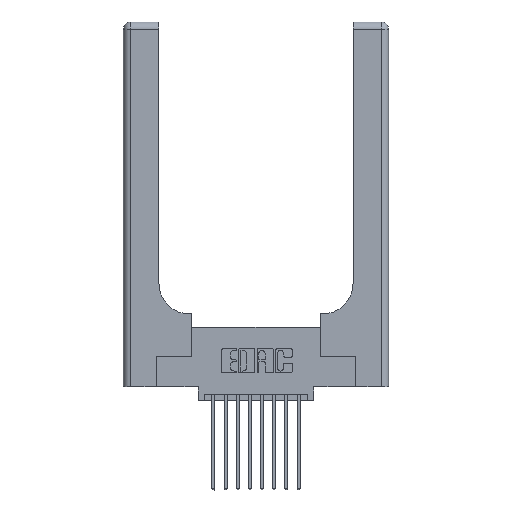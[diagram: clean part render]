
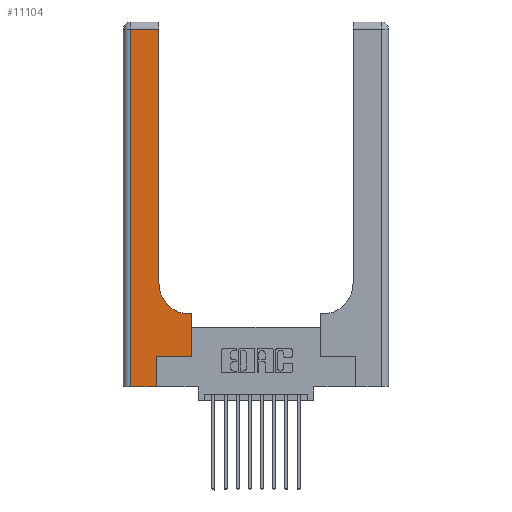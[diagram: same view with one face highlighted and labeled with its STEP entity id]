
A CAD part, top view. The second image highlights one B-rep face of the part: STEP entity #11104.
In plain terms, the highlighted planar face has unit normal (0, 0, 1).
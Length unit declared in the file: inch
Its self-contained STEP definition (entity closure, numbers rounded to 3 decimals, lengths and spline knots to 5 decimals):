
#32 = DIRECTION ( 'NONE',  ( -1., 0., 0. ) ) ;
#150 = DIRECTION ( 'NONE',  ( 0., 1., 0. ) ) ;
#166 = VERTEX_POINT ( 'NONE', #7051 ) ;
#197 = VECTOR ( 'NONE', #150, 39.37008 ) ;
#571 = VERTEX_POINT ( 'NONE', #14026 ) ;
#918 = EDGE_CURVE ( 'NONE', #5515, #571, #5145, .T. ) ;
#1034 = VERTEX_POINT ( 'NONE', #2276 ) ;
#1112 = EDGE_CURVE ( 'NONE', #11790, #7345, #11933, .T. ) ;
#1241 = CARTESIAN_POINT ( 'NONE',  ( 0.2915, 0.6, 0.37 ) ) ;
#1293 = VECTOR ( 'NONE', #6406, 39.37008 ) ;
#1308 = EDGE_CURVE ( 'NONE', #15248, #11790, #1382, .T. ) ;
#1382 = LINE ( 'NONE', #6415, #197 ) ;
#1489 = CARTESIAN_POINT ( 'NONE',  ( 0.5585, 0.25, 0.37 ) ) ;
#1507 = CARTESIAN_POINT ( 'NONE',  ( 0.06, 3., 0.37 ) ) ;
#1772 = AXIS2_PLACEMENT_3D ( 'NONE', #3722, #12436, #4981 ) ;
#1976 = EDGE_CURVE ( 'NONE', #7345, #1034, #12195, .T. ) ;
#2276 = CARTESIAN_POINT ( 'NONE',  ( 0.06, 0., 0.37 ) ) ;
#2328 = ORIENTED_EDGE ( 'NONE', *, *, #5611, .T. ) ;
#2568 = DIRECTION ( 'NONE',  ( -1., 0., 0. ) ) ;
#2602 = VECTOR ( 'NONE', #11619, 39.37008 ) ;
#2832 = CARTESIAN_POINT ( 'NONE',  ( 0., 0., 0.37 ) ) ;
#3722 = CARTESIAN_POINT ( 'NONE',  ( 0.5415, 0.85, 0.37 ) ) ;
#3747 = ORIENTED_EDGE ( 'NONE', *, *, #15463, .T. ) ;
#3814 = ORIENTED_EDGE ( 'NONE', *, *, #13685, .T. ) ;
#4015 = EDGE_LOOP ( 'NONE', ( #8840, #10055, #9862, #3814, #5049, #3747, #7966, #4863, #2328 ) ) ;
#4237 = EDGE_CURVE ( 'NONE', #4382, #5515, #6506, .T. ) ;
#4382 = VERTEX_POINT ( 'NONE', #12484 ) ;
#4863 = ORIENTED_EDGE ( 'NONE', *, *, #918, .T. ) ;
#4981 = DIRECTION ( 'NONE',  ( 1., 0., 0. ) ) ;
#5049 = ORIENTED_EDGE ( 'NONE', *, *, #8707, .T. ) ;
#5053 = FACE_OUTER_BOUND ( 'NONE', #4015, .T. ) ;
#5145 = LINE ( 'NONE', #1241, #13120 ) ;
#5431 = AXIS2_PLACEMENT_3D ( 'NONE', #9838, #6297, #32 ) ;
#5515 = VERTEX_POINT ( 'NONE', #10872 ) ;
#5611 = EDGE_CURVE ( 'NONE', #571, #15248, #5868, .T. ) ;
#5739 = LINE ( 'NONE', #2832, #2602 ) ;
#5868 = CIRCLE ( 'NONE', #1772, 0.25 ) ;
#6297 = DIRECTION ( 'NONE',  ( 0., 0., -1. ) ) ;
#6406 = DIRECTION ( 'NONE',  ( 1., 0., 0. ) ) ;
#6415 = CARTESIAN_POINT ( 'NONE',  ( 0.2915, 3., 0.37 ) ) ;
#6506 = LINE ( 'NONE', #1489, #7053 ) ;
#7051 = CARTESIAN_POINT ( 'NONE',  ( 0.269, 0., 0.37 ) ) ;
#7053 = VECTOR ( 'NONE', #9040, 39.37008 ) ;
#7078 = DIRECTION ( 'NONE',  ( -1., 0., 0. ) ) ;
#7345 = VERTEX_POINT ( 'NONE', #14695 ) ;
#7966 = ORIENTED_EDGE ( 'NONE', *, *, #4237, .T. ) ;
#8199 = CARTESIAN_POINT ( 'NONE',  ( 0.269, 0.25, 0.37 ) ) ;
#8559 = DIRECTION ( 'NONE',  ( 0., 1., 0. ) ) ;
#8707 = EDGE_CURVE ( 'NONE', #166, #15069, #8970, .T. ) ;
#8840 = ORIENTED_EDGE ( 'NONE', *, *, #1308, .T. ) ;
#8970 = LINE ( 'NONE', #15930, #14453 ) ;
#9040 = DIRECTION ( 'NONE',  ( 0., 1., 0. ) ) ;
#9439 = CARTESIAN_POINT ( 'NONE',  ( 0., 2.94, 0.37 ) ) ;
#9657 = VECTOR ( 'NONE', #12991, 39.37008 ) ;
#9838 = CARTESIAN_POINT ( 'NONE',  ( 0., 3., 0.37 ) ) ;
#9841 = CARTESIAN_POINT ( 'NONE',  ( 0.2915, 0.85, 0.37 ) ) ;
#9862 = ORIENTED_EDGE ( 'NONE', *, *, #1976, .T. ) ;
#10055 = ORIENTED_EDGE ( 'NONE', *, *, #1112, .T. ) ;
#10365 = VECTOR ( 'NONE', #7078, 39.37008 ) ;
#10872 = CARTESIAN_POINT ( 'NONE',  ( 0.5585, 0.6, 0.37 ) ) ;
#11104 = ADVANCED_FACE ( 'NONE', ( #5053 ), #12284, .F. ) ;
#11619 = DIRECTION ( 'NONE',  ( 1., 0., 0. ) ) ;
#11790 = VERTEX_POINT ( 'NONE', #15984 ) ;
#11933 = LINE ( 'NONE', #9439, #10365 ) ;
#12195 = LINE ( 'NONE', #1507, #9657 ) ;
#12284 = PLANE ( 'NONE',  #5431 ) ;
#12436 = DIRECTION ( 'NONE',  ( 0., 0., -1. ) ) ;
#12484 = CARTESIAN_POINT ( 'NONE',  ( 0.5585, 0.25, 0.37 ) ) ;
#12991 = DIRECTION ( 'NONE',  ( 0., -1., 0. ) ) ;
#13030 = LINE ( 'NONE', #13880, #1293 ) ;
#13120 = VECTOR ( 'NONE', #2568, 39.37008 ) ;
#13685 = EDGE_CURVE ( 'NONE', #1034, #166, #5739, .T. ) ;
#13880 = CARTESIAN_POINT ( 'NONE',  ( 0.269, 0.25, 0.37 ) ) ;
#14026 = CARTESIAN_POINT ( 'NONE',  ( 0.5415, 0.6, 0.37 ) ) ;
#14453 = VECTOR ( 'NONE', #8559, 39.37008 ) ;
#14695 = CARTESIAN_POINT ( 'NONE',  ( 0.06, 2.94, 0.37 ) ) ;
#15069 = VERTEX_POINT ( 'NONE', #8199 ) ;
#15248 = VERTEX_POINT ( 'NONE', #9841 ) ;
#15463 = EDGE_CURVE ( 'NONE', #15069, #4382, #13030, .T. ) ;
#15930 = CARTESIAN_POINT ( 'NONE',  ( 0.269, 0., 0.37 ) ) ;
#15984 = CARTESIAN_POINT ( 'NONE',  ( 0.2915, 2.94, 0.37 ) ) ;
